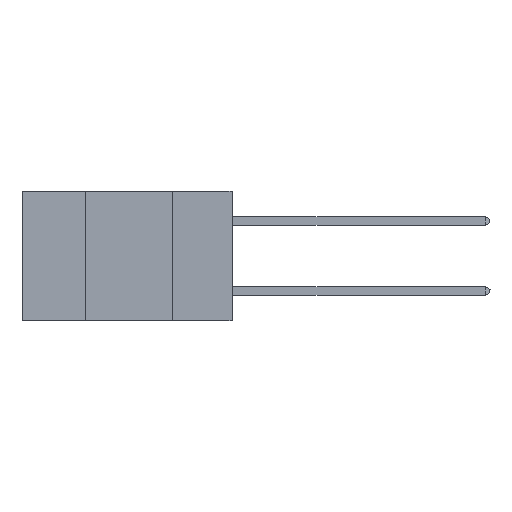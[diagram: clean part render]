
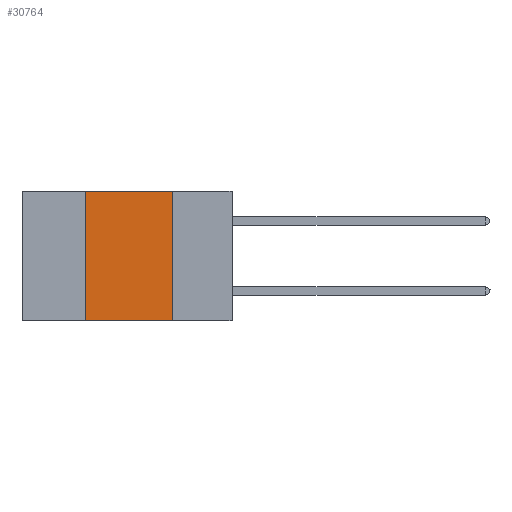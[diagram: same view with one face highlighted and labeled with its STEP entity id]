
A CAD part, left-side view. The second image highlights one B-rep face of the part: STEP entity #30764.
In plain terms, the highlighted planar face has unit normal (-1, 0, 0).
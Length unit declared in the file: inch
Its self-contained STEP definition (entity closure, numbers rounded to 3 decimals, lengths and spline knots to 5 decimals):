
#2503 = DIRECTION ( 'NONE',  ( 0., 0., -1. ) ) ;
#4161 = ORIENTED_EDGE ( 'NONE', *, *, #23830, .T. ) ;
#4533 = CARTESIAN_POINT ( 'NONE',  ( 0., 0.6, -0.37 ) ) ;
#5087 = DIRECTION ( 'NONE',  ( 0., 0., 1. ) ) ;
#5381 = CARTESIAN_POINT ( 'NONE',  ( 0., 0.17, -0.37 ) ) ;
#7056 = CARTESIAN_POINT ( 'NONE',  ( 0., 0.42, 0. ) ) ;
#7889 = CARTESIAN_POINT ( 'NONE',  ( 0., 0.42, -0.37 ) ) ;
#8450 = LINE ( 'NONE', #7056, #27257 ) ;
#8509 = EDGE_CURVE ( 'NONE', #17057, #25113, #8450, .T. ) ;
#8905 = DIRECTION ( 'NONE',  ( 0., -1., 0. ) ) ;
#9257 = LINE ( 'NONE', #4533, #17958 ) ;
#12335 = LINE ( 'NONE', #16691, #18751 ) ;
#12506 = CARTESIAN_POINT ( 'NONE',  ( 0., 0.17, 0. ) ) ;
#13099 = CARTESIAN_POINT ( 'NONE',  ( 0., 0.6, 0. ) ) ;
#13213 = PLANE ( 'NONE',  #22638 ) ;
#14381 = FACE_OUTER_BOUND ( 'NONE', #14567, .T. ) ;
#14567 = EDGE_LOOP ( 'NONE', ( #25319, #17691, #23077, #4161 ) ) ;
#15520 = DIRECTION ( 'NONE',  ( 0., 0., -1. ) ) ;
#16691 = CARTESIAN_POINT ( 'NONE',  ( 0., 0.17, 0. ) ) ;
#17057 = VERTEX_POINT ( 'NONE', #7889 ) ;
#17384 = EDGE_CURVE ( 'NONE', #25113, #25309, #28236, .T. ) ;
#17691 = ORIENTED_EDGE ( 'NONE', *, *, #17384, .F. ) ;
#17958 = VECTOR ( 'NONE', #8905, 39.37008 ) ;
#18147 = VECTOR ( 'NONE', #30725, 39.37008 ) ;
#18161 = DIRECTION ( 'NONE',  ( 1., 0., 0. ) ) ;
#18460 = CARTESIAN_POINT ( 'NONE',  ( 0., 0.42, 0. ) ) ;
#18751 = VECTOR ( 'NONE', #2503, 39.37008 ) ;
#18908 = CARTESIAN_POINT ( 'NONE',  ( 0., 0.6, 0. ) ) ;
#22221 = VERTEX_POINT ( 'NONE', #5381 ) ;
#22638 = AXIS2_PLACEMENT_3D ( 'NONE', #13099, #18161, #15520 ) ;
#23077 = ORIENTED_EDGE ( 'NONE', *, *, #8509, .F. ) ;
#23830 = EDGE_CURVE ( 'NONE', #17057, #22221, #9257, .T. ) ;
#25113 = VERTEX_POINT ( 'NONE', #18460 ) ;
#25309 = VERTEX_POINT ( 'NONE', #12506 ) ;
#25319 = ORIENTED_EDGE ( 'NONE', *, *, #27236, .F. ) ;
#27236 = EDGE_CURVE ( 'NONE', #25309, #22221, #12335, .T. ) ;
#27257 = VECTOR ( 'NONE', #5087, 39.37008 ) ;
#28236 = LINE ( 'NONE', #18908, #18147 ) ;
#30725 = DIRECTION ( 'NONE',  ( 0., -1., 0. ) ) ;
#30764 = ADVANCED_FACE ( 'NONE', ( #14381 ), #13213, .F. ) ;
